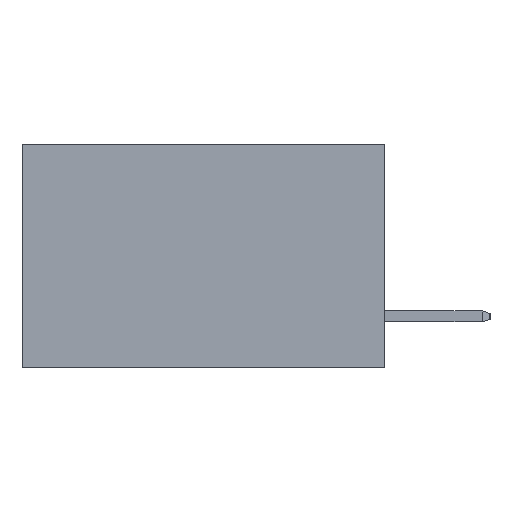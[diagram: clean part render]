
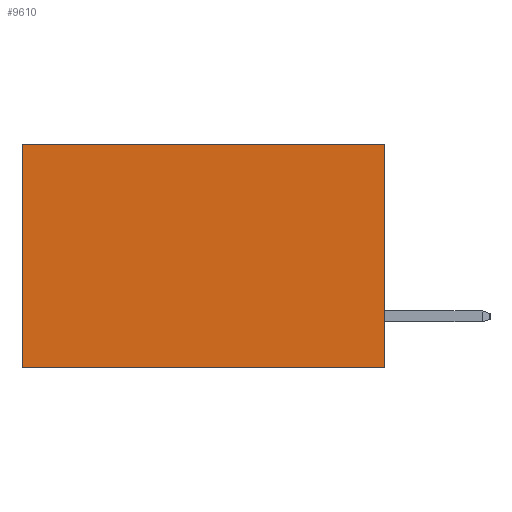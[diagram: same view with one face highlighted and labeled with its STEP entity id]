
A CAD part, left-side view. The second image highlights one B-rep face of the part: STEP entity #9610.
In plain terms, the highlighted planar face has unit normal (-1, 0, 0).
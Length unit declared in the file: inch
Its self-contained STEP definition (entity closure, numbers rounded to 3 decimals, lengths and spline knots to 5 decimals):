
#1050 = DIRECTION ( 'NONE',  ( 0., 0., -1. ) ) ;
#1052 = DIRECTION ( 'NONE',  ( 1., 0., 0. ) ) ;
#1077 = CARTESIAN_POINT ( 'NONE',  ( 0.2615, 0., -0.37 ) ) ;
#1204 = PLANE ( 'NONE',  #19170 ) ;
#2021 = LINE ( 'NONE', #20985, #5994 ) ;
#3279 = LINE ( 'NONE', #14077, #11673 ) ;
#4102 = EDGE_CURVE ( 'NONE', #17413, #13113, #14447, .T. ) ;
#5253 = DIRECTION ( 'NONE',  ( 0., 1., 0. ) ) ;
#5334 = VERTEX_POINT ( 'NONE', #21023 ) ;
#5348 = EDGE_CURVE ( 'NONE', #5334, #17413, #2021, .T. ) ;
#5697 = LINE ( 'NONE', #18659, #18493 ) ;
#5994 = VECTOR ( 'NONE', #20778, 39.37008 ) ;
#6641 = ORIENTED_EDGE ( 'NONE', *, *, #8498, .T. ) ;
#6848 = CARTESIAN_POINT ( 'NONE',  ( 0.2615, 0., -0.37 ) ) ;
#7658 = EDGE_LOOP ( 'NONE', ( #6641, #7701, #19512, #11932 ) ) ;
#7701 = ORIENTED_EDGE ( 'NONE', *, *, #4102, .F. ) ;
#8105 = VERTEX_POINT ( 'NONE', #19613 ) ;
#8153 = EDGE_CURVE ( 'NONE', #5334, #8105, #5697, .T. ) ;
#8498 = EDGE_CURVE ( 'NONE', #8105, #13113, #3279, .T. ) ;
#9610 = ADVANCED_FACE ( 'NONE', ( #15042 ), #1204, .F. ) ;
#11673 = VECTOR ( 'NONE', #14108, 39.37008 ) ;
#11932 = ORIENTED_EDGE ( 'NONE', *, *, #8153, .T. ) ;
#13113 = VERTEX_POINT ( 'NONE', #15743 ) ;
#14077 = CARTESIAN_POINT ( 'NONE',  ( 0.2615, 0.6, -0.37 ) ) ;
#14108 = DIRECTION ( 'NONE',  ( 0., 0., -1. ) ) ;
#14447 = LINE ( 'NONE', #6848, #18361 ) ;
#15042 = FACE_OUTER_BOUND ( 'NONE', #7658, .T. ) ;
#15743 = CARTESIAN_POINT ( 'NONE',  ( 0.2615, 0.6, -0.37 ) ) ;
#17413 = VERTEX_POINT ( 'NONE', #21548 ) ;
#18361 = VECTOR ( 'NONE', #5253, 39.37008 ) ;
#18493 = VECTOR ( 'NONE', #19053, 39.37008 ) ;
#18659 = CARTESIAN_POINT ( 'NONE',  ( 0.2615, 0., 0. ) ) ;
#19053 = DIRECTION ( 'NONE',  ( 0., 1., 0. ) ) ;
#19170 = AXIS2_PLACEMENT_3D ( 'NONE', #1077, #1052, #1050 ) ;
#19512 = ORIENTED_EDGE ( 'NONE', *, *, #5348, .F. ) ;
#19613 = CARTESIAN_POINT ( 'NONE',  ( 0.2615, 0.6, 0. ) ) ;
#20778 = DIRECTION ( 'NONE',  ( 0., 0., -1. ) ) ;
#20985 = CARTESIAN_POINT ( 'NONE',  ( 0.2615, 0., -0.37 ) ) ;
#21023 = CARTESIAN_POINT ( 'NONE',  ( 0.2615, 0., 0. ) ) ;
#21548 = CARTESIAN_POINT ( 'NONE',  ( 0.2615, 0., -0.37 ) ) ;
